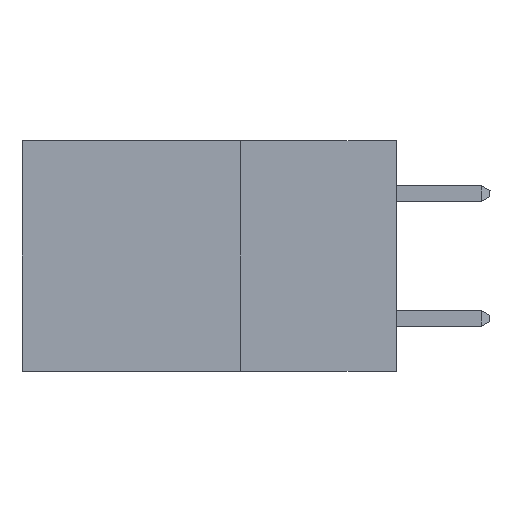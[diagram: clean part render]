
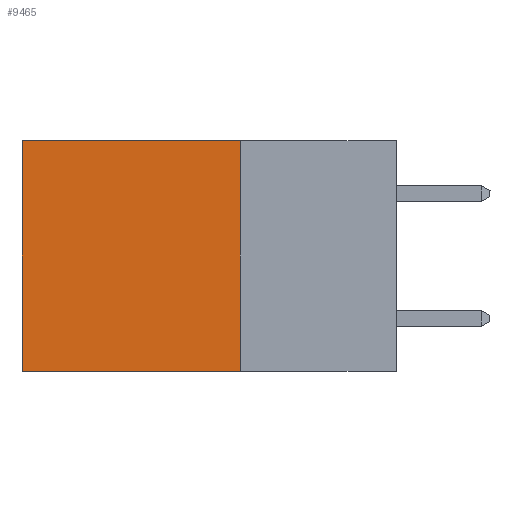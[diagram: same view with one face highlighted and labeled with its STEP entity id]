
A CAD part, left-side view. The second image highlights one B-rep face of the part: STEP entity #9465.
In plain terms, the highlighted planar face has unit normal (-1, 0, 0).
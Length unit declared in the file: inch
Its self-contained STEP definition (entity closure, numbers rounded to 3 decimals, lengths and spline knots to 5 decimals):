
#896 = ORIENTED_EDGE ( 'NONE', *, *, #5785, .F. ) ;
#1130 = EDGE_CURVE ( 'NONE', #3287, #8335, #3101, .T. ) ;
#1326 = CARTESIAN_POINT ( 'NONE',  ( 0.298, 0.25, -0.37 ) ) ;
#1540 = ORIENTED_EDGE ( 'NONE', *, *, #1130, .F. ) ;
#1600 = CARTESIAN_POINT ( 'NONE',  ( 0.298, 0.6, 0. ) ) ;
#1626 = EDGE_LOOP ( 'NONE', ( #9283, #896, #1540, #13987 ) ) ;
#2125 = VERTEX_POINT ( 'NONE', #1600 ) ;
#2458 = DIRECTION ( 'NONE',  ( 0., 0., -1. ) ) ;
#2891 = VECTOR ( 'NONE', #10792, 39.37008 ) ;
#3094 = PLANE ( 'NONE',  #6726 ) ;
#3101 = LINE ( 'NONE', #6117, #3482 ) ;
#3287 = VERTEX_POINT ( 'NONE', #11402 ) ;
#3438 = LINE ( 'NONE', #9301, #9184 ) ;
#3448 = EDGE_CURVE ( 'NONE', #3287, #2125, #12002, .T. ) ;
#3482 = VECTOR ( 'NONE', #6076, 39.37008 ) ;
#5785 = EDGE_CURVE ( 'NONE', #8335, #7092, #11026, .T. ) ;
#6076 = DIRECTION ( 'NONE',  ( 0., 0., -1. ) ) ;
#6117 = CARTESIAN_POINT ( 'NONE',  ( 0.298, 0.25, 0. ) ) ;
#6726 = AXIS2_PLACEMENT_3D ( 'NONE', #11048, #14562, #7709 ) ;
#7092 = VERTEX_POINT ( 'NONE', #10809 ) ;
#7709 = DIRECTION ( 'NONE',  ( 0., 0., -1. ) ) ;
#8335 = VERTEX_POINT ( 'NONE', #14856 ) ;
#8427 = EDGE_CURVE ( 'NONE', #2125, #7092, #3438, .T. ) ;
#9184 = VECTOR ( 'NONE', #2458, 39.37008 ) ;
#9283 = ORIENTED_EDGE ( 'NONE', *, *, #8427, .T. ) ;
#9301 = CARTESIAN_POINT ( 'NONE',  ( 0.298, 0.6, 0. ) ) ;
#9465 = ADVANCED_FACE ( 'NONE', ( #10020 ), #3094, .F. ) ;
#10020 = FACE_OUTER_BOUND ( 'NONE', #1626, .T. ) ;
#10669 = VECTOR ( 'NONE', #13054, 39.37008 ) ;
#10792 = DIRECTION ( 'NONE',  ( 0., 1., 0. ) ) ;
#10809 = CARTESIAN_POINT ( 'NONE',  ( 0.298, 0.6, -0.37 ) ) ;
#11026 = LINE ( 'NONE', #1326, #10669 ) ;
#11048 = CARTESIAN_POINT ( 'NONE',  ( 0.298, 0.25, 0. ) ) ;
#11402 = CARTESIAN_POINT ( 'NONE',  ( 0.298, 0.25, 0. ) ) ;
#11860 = CARTESIAN_POINT ( 'NONE',  ( 0.298, 0.25, 0. ) ) ;
#12002 = LINE ( 'NONE', #11860, #2891 ) ;
#13054 = DIRECTION ( 'NONE',  ( 0., 1., 0. ) ) ;
#13987 = ORIENTED_EDGE ( 'NONE', *, *, #3448, .T. ) ;
#14562 = DIRECTION ( 'NONE',  ( 1., 0., 0. ) ) ;
#14856 = CARTESIAN_POINT ( 'NONE',  ( 0.298, 0.25, -0.37 ) ) ;
